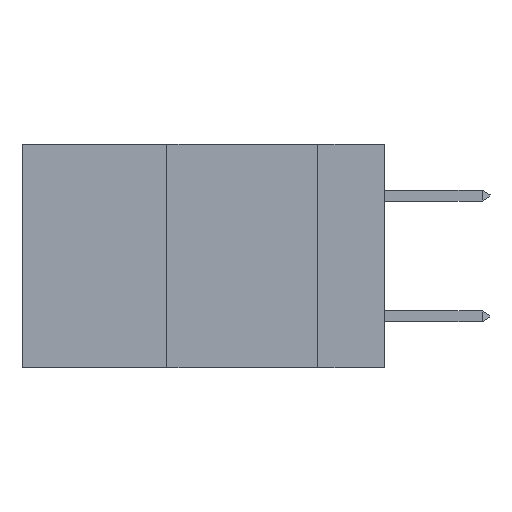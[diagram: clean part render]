
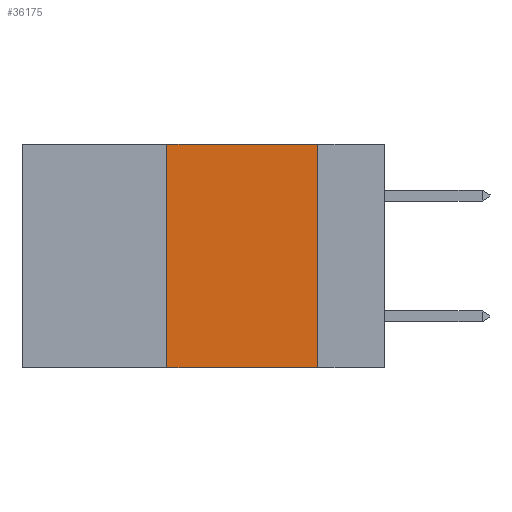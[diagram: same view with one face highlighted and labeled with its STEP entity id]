
A CAD part, left-side view. The second image highlights one B-rep face of the part: STEP entity #36175.
In plain terms, the highlighted planar face has unit normal (-1, 0, 0).
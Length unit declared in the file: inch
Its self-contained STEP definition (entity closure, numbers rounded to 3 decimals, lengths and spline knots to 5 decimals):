
#649 = CARTESIAN_POINT ( 'NONE',  ( 0., 0.6, 0. ) ) ;
#759 = ORIENTED_EDGE ( 'NONE', *, *, #21310, .F. ) ;
#966 = EDGE_LOOP ( 'NONE', ( #6549, #759, #20067, #25241 ) ) ;
#3708 = CARTESIAN_POINT ( 'NONE',  ( 0., 0.6, 0. ) ) ;
#4306 = CARTESIAN_POINT ( 'NONE',  ( 0., 0.6, -0.37 ) ) ;
#4408 = CARTESIAN_POINT ( 'NONE',  ( 0., 0.36, 0. ) ) ;
#4539 = CARTESIAN_POINT ( 'NONE',  ( 0., 0.11, 0. ) ) ;
#5556 = LINE ( 'NONE', #13413, #28406 ) ;
#6058 = VERTEX_POINT ( 'NONE', #4408 ) ;
#6549 = ORIENTED_EDGE ( 'NONE', *, *, #24964, .F. ) ;
#8274 = EDGE_CURVE ( 'NONE', #25971, #6058, #5556, .T. ) ;
#9259 = DIRECTION ( 'NONE',  ( 1., 0., 0. ) ) ;
#10347 = VERTEX_POINT ( 'NONE', #24870 ) ;
#10405 = DIRECTION ( 'NONE',  ( 0., 0., -1. ) ) ;
#10946 = CARTESIAN_POINT ( 'NONE',  ( 0., 0.36, -0.37 ) ) ;
#11905 = PLANE ( 'NONE',  #12285 ) ;
#12285 = AXIS2_PLACEMENT_3D ( 'NONE', #649, #9259, #15642 ) ;
#12705 = VERTEX_POINT ( 'NONE', #18976 ) ;
#13084 = LINE ( 'NONE', #3708, #25622 ) ;
#13413 = CARTESIAN_POINT ( 'NONE',  ( 0., 0.36, 0. ) ) ;
#15642 = DIRECTION ( 'NONE',  ( 0., 0., -1. ) ) ;
#15682 = DIRECTION ( 'NONE',  ( 0., -1., 0. ) ) ;
#17546 = FACE_OUTER_BOUND ( 'NONE', #966, .T. ) ;
#18976 = CARTESIAN_POINT ( 'NONE',  ( 0., 0.11, 0. ) ) ;
#20067 = ORIENTED_EDGE ( 'NONE', *, *, #8274, .F. ) ;
#20833 = LINE ( 'NONE', #4539, #35189 ) ;
#21310 = EDGE_CURVE ( 'NONE', #6058, #12705, #13084, .T. ) ;
#21359 = DIRECTION ( 'NONE',  ( 0., -1., 0. ) ) ;
#22619 = LINE ( 'NONE', #4306, #36502 ) ;
#22797 = EDGE_CURVE ( 'NONE', #25971, #10347, #22619, .T. ) ;
#24870 = CARTESIAN_POINT ( 'NONE',  ( 0., 0.11, -0.37 ) ) ;
#24964 = EDGE_CURVE ( 'NONE', #12705, #10347, #20833, .T. ) ;
#25241 = ORIENTED_EDGE ( 'NONE', *, *, #22797, .T. ) ;
#25622 = VECTOR ( 'NONE', #21359, 39.37008 ) ;
#25971 = VERTEX_POINT ( 'NONE', #10946 ) ;
#27560 = DIRECTION ( 'NONE',  ( 0., 0., 1. ) ) ;
#28406 = VECTOR ( 'NONE', #27560, 39.37008 ) ;
#35189 = VECTOR ( 'NONE', #10405, 39.37008 ) ;
#36175 = ADVANCED_FACE ( 'NONE', ( #17546 ), #11905, .F. ) ;
#36502 = VECTOR ( 'NONE', #15682, 39.37008 ) ;
